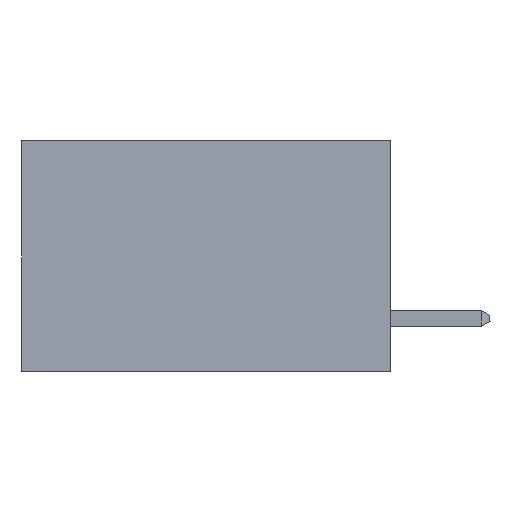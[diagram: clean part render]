
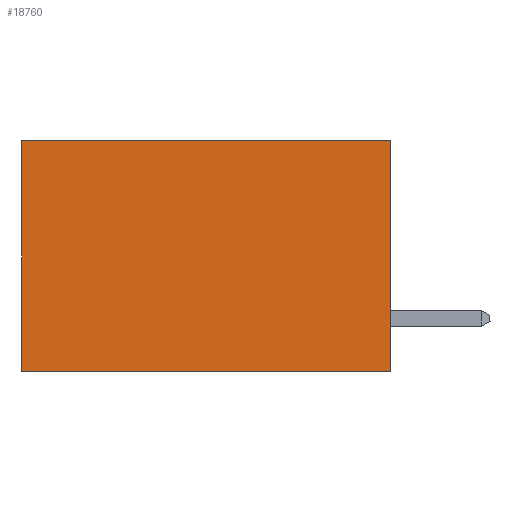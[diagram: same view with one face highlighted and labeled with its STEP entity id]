
A CAD part, left-side view. The second image highlights one B-rep face of the part: STEP entity #18760.
In plain terms, the highlighted planar face has unit normal (-1, 0, 0).
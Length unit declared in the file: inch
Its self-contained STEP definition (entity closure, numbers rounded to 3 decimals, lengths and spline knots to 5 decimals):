
#315 = CARTESIAN_POINT ( 'NONE',  ( 0.277, 0., 0. ) ) ;
#342 = LINE ( 'NONE', #13220, #5083 ) ;
#1591 = CARTESIAN_POINT ( 'NONE',  ( 0.277, 0., -0.37 ) ) ;
#1973 = LINE ( 'NONE', #12483, #19860 ) ;
#3072 = VERTEX_POINT ( 'NONE', #7443 ) ;
#3246 = PLANE ( 'NONE',  #15963 ) ;
#4204 = CARTESIAN_POINT ( 'NONE',  ( 0.277, 0.59, 0. ) ) ;
#4335 = FACE_OUTER_BOUND ( 'NONE', #10665, .T. ) ;
#4504 = ORIENTED_EDGE ( 'NONE', *, *, #15649, .T. ) ;
#5083 = VECTOR ( 'NONE', #14970, 39.37008 ) ;
#6812 = DIRECTION ( 'NONE',  ( 1., 0., 0. ) ) ;
#6870 = EDGE_CURVE ( 'NONE', #20364, #3072, #14770, .T. ) ;
#7307 = DIRECTION ( 'NONE',  ( 0., 1., 0. ) ) ;
#7443 = CARTESIAN_POINT ( 'NONE',  ( 0.277, 0.59, -0.37 ) ) ;
#7565 = CARTESIAN_POINT ( 'NONE',  ( 0.277, 0., -0.37 ) ) ;
#8699 = VERTEX_POINT ( 'NONE', #315 ) ;
#10117 = VECTOR ( 'NONE', #11058, 39.37008 ) ;
#10411 = EDGE_CURVE ( 'NONE', #8699, #20364, #20468, .T. ) ;
#10665 = EDGE_LOOP ( 'NONE', ( #11163, #12069, #18501, #4504 ) ) ;
#11058 = DIRECTION ( 'NONE',  ( 0., 1., 0. ) ) ;
#11110 = CARTESIAN_POINT ( 'NONE',  ( 0.277, 0., -0.37 ) ) ;
#11163 = ORIENTED_EDGE ( 'NONE', *, *, #14628, .T. ) ;
#12069 = ORIENTED_EDGE ( 'NONE', *, *, #6870, .F. ) ;
#12073 = DIRECTION ( 'NONE',  ( 0., 0., -1. ) ) ;
#12483 = CARTESIAN_POINT ( 'NONE',  ( 0.277, 0., 0. ) ) ;
#13220 = CARTESIAN_POINT ( 'NONE',  ( 0.277, 0.59, -0.37 ) ) ;
#14628 = EDGE_CURVE ( 'NONE', #18453, #3072, #342, .T. ) ;
#14770 = LINE ( 'NONE', #11110, #10117 ) ;
#14970 = DIRECTION ( 'NONE',  ( 0., 0., -1. ) ) ;
#15649 = EDGE_CURVE ( 'NONE', #8699, #18453, #1973, .T. ) ;
#15963 = AXIS2_PLACEMENT_3D ( 'NONE', #17185, #6812, #18873 ) ;
#17185 = CARTESIAN_POINT ( 'NONE',  ( 0.277, 0., -0.37 ) ) ;
#18453 = VERTEX_POINT ( 'NONE', #4204 ) ;
#18501 = ORIENTED_EDGE ( 'NONE', *, *, #10411, .F. ) ;
#18760 = ADVANCED_FACE ( 'NONE', ( #4335 ), #3246, .F. ) ;
#18873 = DIRECTION ( 'NONE',  ( 0., 0., -1. ) ) ;
#19860 = VECTOR ( 'NONE', #7307, 39.37008 ) ;
#19954 = VECTOR ( 'NONE', #12073, 39.37008 ) ;
#20364 = VERTEX_POINT ( 'NONE', #7565 ) ;
#20468 = LINE ( 'NONE', #1591, #19954 ) ;
